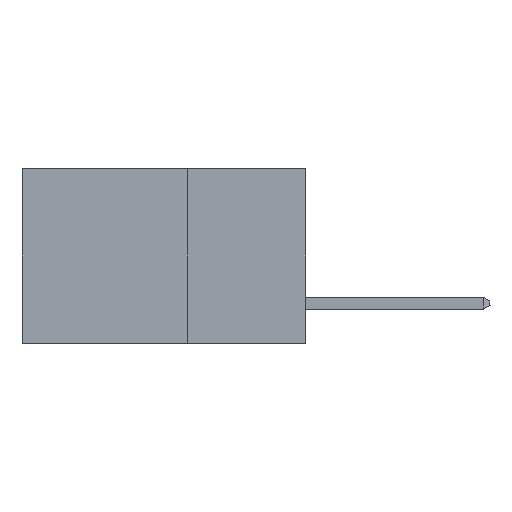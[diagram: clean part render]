
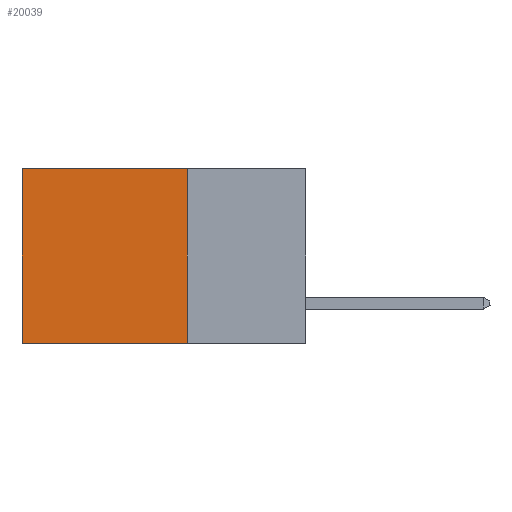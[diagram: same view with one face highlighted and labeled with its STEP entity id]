
A CAD part, left-side view. The second image highlights one B-rep face of the part: STEP entity #20039.
In plain terms, the highlighted planar face has unit normal (-1, 0, 0).
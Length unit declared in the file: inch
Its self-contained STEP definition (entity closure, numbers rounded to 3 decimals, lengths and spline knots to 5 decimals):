
#21 = CARTESIAN_POINT ( 'NONE',  ( 0.298, 0.25, 0. ) ) ;
#828 = ORIENTED_EDGE ( 'NONE', *, *, #13765, .T. ) ;
#1311 = VECTOR ( 'NONE', #19796, 39.37008 ) ;
#1684 = DIRECTION ( 'NONE',  ( 0., 0., -1. ) ) ;
#1693 = ORIENTED_EDGE ( 'NONE', *, *, #20524, .T. ) ;
#1843 = FACE_OUTER_BOUND ( 'NONE', #21637, .T. ) ;
#2911 = CARTESIAN_POINT ( 'NONE',  ( 0.298, 0.25, 0. ) ) ;
#6866 = ORIENTED_EDGE ( 'NONE', *, *, #13595, .F. ) ;
#6951 = AXIS2_PLACEMENT_3D ( 'NONE', #13161, #15193, #8720 ) ;
#8720 = DIRECTION ( 'NONE',  ( 0., 0., -1. ) ) ;
#10086 = CARTESIAN_POINT ( 'NONE',  ( 0.298, 0.25, -0.37 ) ) ;
#11465 = EDGE_CURVE ( 'NONE', #13527, #17724, #20942, .T. ) ;
#12349 = CARTESIAN_POINT ( 'NONE',  ( 0.298, 0.6, -0.37 ) ) ;
#13161 = CARTESIAN_POINT ( 'NONE',  ( 0.298, 0.25, 0. ) ) ;
#13527 = VERTEX_POINT ( 'NONE', #21 ) ;
#13595 = EDGE_CURVE ( 'NONE', #17724, #24863, #25540, .T. ) ;
#13765 = EDGE_CURVE ( 'NONE', #13527, #21217, #13924, .T. ) ;
#13924 = LINE ( 'NONE', #2911, #1311 ) ;
#15193 = DIRECTION ( 'NONE',  ( 1., 0., 0. ) ) ;
#15417 = CARTESIAN_POINT ( 'NONE',  ( 0.298, 0.25, -0.37 ) ) ;
#15734 = VECTOR ( 'NONE', #21277, 39.37008 ) ;
#16240 = VECTOR ( 'NONE', #26005, 39.37008 ) ;
#16616 = VECTOR ( 'NONE', #1684, 39.37008 ) ;
#17247 = PLANE ( 'NONE',  #6951 ) ;
#17724 = VERTEX_POINT ( 'NONE', #10086 ) ;
#18460 = CARTESIAN_POINT ( 'NONE',  ( 0.298, 0.25, 0. ) ) ;
#19796 = DIRECTION ( 'NONE',  ( 0., 1., 0. ) ) ;
#20039 = ADVANCED_FACE ( 'NONE', ( #1843 ), #17247, .F. ) ;
#20524 = EDGE_CURVE ( 'NONE', #21217, #24863, #25042, .T. ) ;
#20942 = LINE ( 'NONE', #18460, #16616 ) ;
#21217 = VERTEX_POINT ( 'NONE', #26530 ) ;
#21277 = DIRECTION ( 'NONE',  ( 0., 0., -1. ) ) ;
#21637 = EDGE_LOOP ( 'NONE', ( #1693, #6866, #23109, #828 ) ) ;
#23109 = ORIENTED_EDGE ( 'NONE', *, *, #11465, .F. ) ;
#24863 = VERTEX_POINT ( 'NONE', #12349 ) ;
#25042 = LINE ( 'NONE', #27406, #15734 ) ;
#25540 = LINE ( 'NONE', #15417, #16240 ) ;
#26005 = DIRECTION ( 'NONE',  ( 0., 1., 0. ) ) ;
#26530 = CARTESIAN_POINT ( 'NONE',  ( 0.298, 0.6, 0. ) ) ;
#27406 = CARTESIAN_POINT ( 'NONE',  ( 0.298, 0.6, 0. ) ) ;
